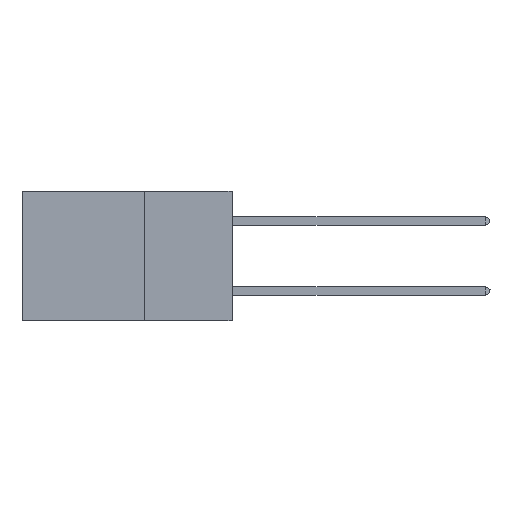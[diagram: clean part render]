
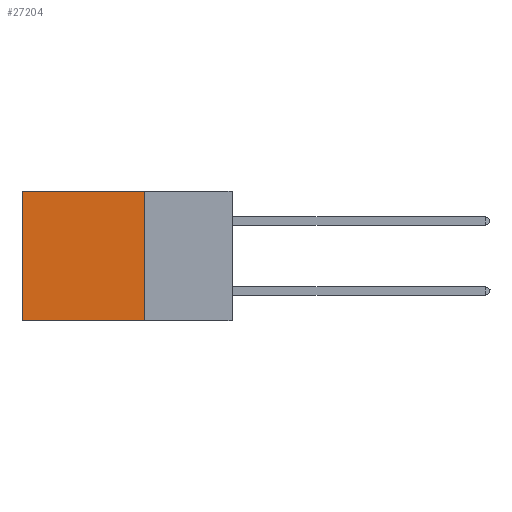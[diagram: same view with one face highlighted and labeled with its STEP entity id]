
A CAD part, left-side view. The second image highlights one B-rep face of the part: STEP entity #27204.
In plain terms, the highlighted planar face has unit normal (-1, 0, 0).
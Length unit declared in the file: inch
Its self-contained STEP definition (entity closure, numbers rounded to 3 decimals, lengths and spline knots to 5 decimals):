
#278 = CARTESIAN_POINT ( 'NONE',  ( 0.2875, 0.6, -0.37 ) ) ;
#310 = CARTESIAN_POINT ( 'NONE',  ( 0.2875, 0.6, 0. ) ) ;
#642 = ORIENTED_EDGE ( 'NONE', *, *, #16755, .T. ) ;
#2740 = VERTEX_POINT ( 'NONE', #278 ) ;
#3910 = CARTESIAN_POINT ( 'NONE',  ( 0.2875, 0.25, 0. ) ) ;
#4320 = EDGE_CURVE ( 'NONE', #26909, #15512, #23981, .T. ) ;
#4894 = VECTOR ( 'NONE', #16223, 39.37008 ) ;
#5666 = VERTEX_POINT ( 'NONE', #310 ) ;
#5776 = LINE ( 'NONE', #12041, #4894 ) ;
#6115 = ORIENTED_EDGE ( 'NONE', *, *, #21048, .F. ) ;
#6348 = LINE ( 'NONE', #10652, #7504 ) ;
#7115 = ORIENTED_EDGE ( 'NONE', *, *, #25676, .T. ) ;
#7504 = VECTOR ( 'NONE', #19191, 39.37008 ) ;
#8097 = PLANE ( 'NONE',  #12101 ) ;
#8364 = DIRECTION ( 'NONE',  ( 1., 0., 0. ) ) ;
#8670 = CARTESIAN_POINT ( 'NONE',  ( 0.2875, 0.25, 0. ) ) ;
#9969 = ORIENTED_EDGE ( 'NONE', *, *, #4320, .F. ) ;
#10313 = DIRECTION ( 'NONE',  ( 0., 0., -1. ) ) ;
#10652 = CARTESIAN_POINT ( 'NONE',  ( 0.2875, 0.6, 0. ) ) ;
#12041 = CARTESIAN_POINT ( 'NONE',  ( 0.2875, 0.25, -0.37 ) ) ;
#12101 = AXIS2_PLACEMENT_3D ( 'NONE', #3910, #8364, #10313 ) ;
#13356 = DIRECTION ( 'NONE',  ( 0., 0., -1. ) ) ;
#14051 = LINE ( 'NONE', #24816, #24964 ) ;
#15512 = VERTEX_POINT ( 'NONE', #23048 ) ;
#16223 = DIRECTION ( 'NONE',  ( 0., 1., 0. ) ) ;
#16718 = FACE_OUTER_BOUND ( 'NONE', #21094, .T. ) ;
#16755 = EDGE_CURVE ( 'NONE', #5666, #2740, #6348, .T. ) ;
#18226 = VECTOR ( 'NONE', #13356, 39.37008 ) ;
#19191 = DIRECTION ( 'NONE',  ( 0., 0., -1. ) ) ;
#20363 = DIRECTION ( 'NONE',  ( 0., 1., 0. ) ) ;
#21048 = EDGE_CURVE ( 'NONE', #15512, #2740, #5776, .T. ) ;
#21094 = EDGE_LOOP ( 'NONE', ( #642, #6115, #9969, #7115 ) ) ;
#23048 = CARTESIAN_POINT ( 'NONE',  ( 0.2875, 0.25, -0.37 ) ) ;
#23981 = LINE ( 'NONE', #26359, #18226 ) ;
#24816 = CARTESIAN_POINT ( 'NONE',  ( 0.2875, 0.25, 0. ) ) ;
#24964 = VECTOR ( 'NONE', #20363, 39.37008 ) ;
#25676 = EDGE_CURVE ( 'NONE', #26909, #5666, #14051, .T. ) ;
#26359 = CARTESIAN_POINT ( 'NONE',  ( 0.2875, 0.25, 0. ) ) ;
#26909 = VERTEX_POINT ( 'NONE', #8670 ) ;
#27204 = ADVANCED_FACE ( 'NONE', ( #16718 ), #8097, .F. ) ;
